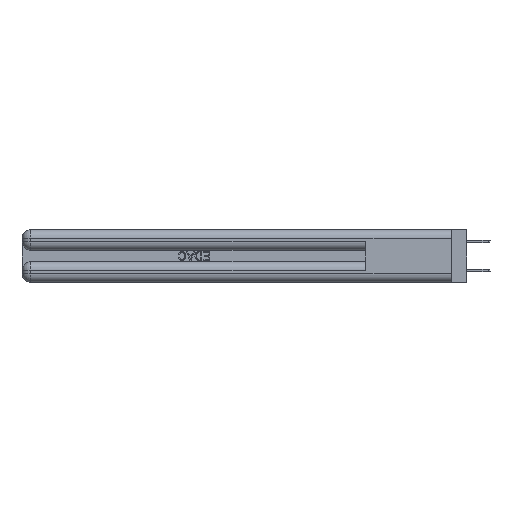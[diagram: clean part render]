
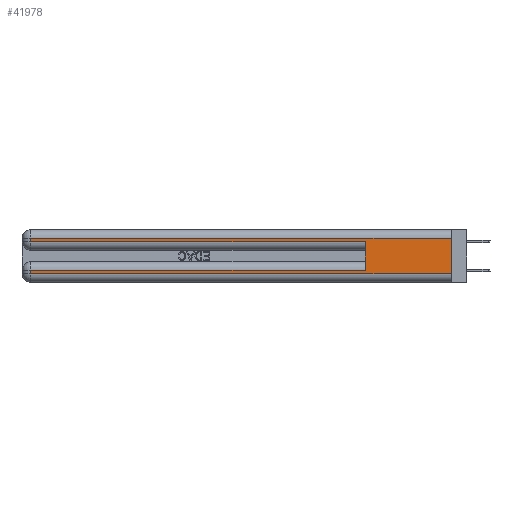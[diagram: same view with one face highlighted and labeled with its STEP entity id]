
A CAD part, left-side view. The second image highlights one B-rep face of the part: STEP entity #41978.
In plain terms, the highlighted planar face has unit normal (-1, 0, 0).
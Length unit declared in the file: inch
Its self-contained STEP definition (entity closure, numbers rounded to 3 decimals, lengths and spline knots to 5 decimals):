
#437 = DIRECTION ( 'NONE',  ( 0., 1., 0. ) ) ;
#550 = EDGE_CURVE ( 'NONE', #6409, #12220, #38957, .T. ) ;
#805 = LINE ( 'NONE', #17639, #45307 ) ;
#3940 = VECTOR ( 'NONE', #19840, 39.37008 ) ;
#4874 = CARTESIAN_POINT ( 'NONE',  ( 0., 0., 0.06 ) ) ;
#4940 = FACE_OUTER_BOUND ( 'NONE', #13955, .T. ) ;
#5453 = ORIENTED_EDGE ( 'NONE', *, *, #22547, .F. ) ;
#5785 = LINE ( 'NONE', #35403, #41984 ) ;
#6293 = DIRECTION ( 'NONE',  ( 0., 1., 0. ) ) ;
#6409 = VERTEX_POINT ( 'NONE', #10281 ) ;
#7810 = VERTEX_POINT ( 'NONE', #4874 ) ;
#7811 = PLANE ( 'NONE',  #12736 ) ;
#8340 = EDGE_CURVE ( 'NONE', #20547, #34211, #5785, .T. ) ;
#8510 = ORIENTED_EDGE ( 'NONE', *, *, #25732, .T. ) ;
#9078 = VERTEX_POINT ( 'NONE', #32416 ) ;
#9186 = LINE ( 'NONE', #11735, #33883 ) ;
#9234 = EDGE_CURVE ( 'NONE', #9078, #27472, #27751, .T. ) ;
#9552 = VECTOR ( 'NONE', #19166, 39.37008 ) ;
#10281 = CARTESIAN_POINT ( 'NONE',  ( 0., 0.6, 0.085 ) ) ;
#11735 = CARTESIAN_POINT ( 'NONE',  ( 0., 2.94, 0.37 ) ) ;
#12220 = VERTEX_POINT ( 'NONE', #26976 ) ;
#12345 = ORIENTED_EDGE ( 'NONE', *, *, #8340, .T. ) ;
#12736 = AXIS2_PLACEMENT_3D ( 'NONE', #14619, #39388, #18491 ) ;
#13955 = EDGE_LOOP ( 'NONE', ( #5453, #12345, #8510, #20647, #45182, #41907, #17926, #29409 ) ) ;
#14619 = CARTESIAN_POINT ( 'NONE',  ( 0., 0., 0.37 ) ) ;
#15609 = CARTESIAN_POINT ( 'NONE',  ( 0., 2.94, 0.37 ) ) ;
#17639 = CARTESIAN_POINT ( 'NONE',  ( 0., 0., 0.06 ) ) ;
#17926 = ORIENTED_EDGE ( 'NONE', *, *, #36855, .T. ) ;
#18491 = DIRECTION ( 'NONE',  ( 0., 0., -1. ) ) ;
#18560 = CARTESIAN_POINT ( 'NONE',  ( 0., 0., 0.37 ) ) ;
#19166 = DIRECTION ( 'NONE',  ( 0., 0., -1. ) ) ;
#19306 = DIRECTION ( 'NONE',  ( 0., -1., 0. ) ) ;
#19840 = DIRECTION ( 'NONE',  ( 0., 0., 1. ) ) ;
#20403 = VECTOR ( 'NONE', #6293, 39.37008 ) ;
#20459 = EDGE_CURVE ( 'NONE', #44820, #7810, #805, .T. ) ;
#20547 = VERTEX_POINT ( 'NONE', #21607 ) ;
#20647 = ORIENTED_EDGE ( 'NONE', *, *, #9234, .T. ) ;
#21158 = DIRECTION ( 'NONE',  ( 0., -1., 0. ) ) ;
#21528 = CARTESIAN_POINT ( 'NONE',  ( 0., 2.94, 0.06 ) ) ;
#21607 = CARTESIAN_POINT ( 'NONE',  ( 0., 0., 0.31 ) ) ;
#22547 = EDGE_CURVE ( 'NONE', #20547, #7810, #44561, .T. ) ;
#24910 = VECTOR ( 'NONE', #35960, 39.37008 ) ;
#25049 = CARTESIAN_POINT ( 'NONE',  ( 0., 0.6, 0.285 ) ) ;
#25732 = EDGE_CURVE ( 'NONE', #34211, #9078, #9186, .T. ) ;
#26976 = CARTESIAN_POINT ( 'NONE',  ( 0., 2.94, 0.085 ) ) ;
#27351 = CARTESIAN_POINT ( 'NONE',  ( 0., 0., 0.085 ) ) ;
#27472 = VERTEX_POINT ( 'NONE', #25049 ) ;
#27751 = LINE ( 'NONE', #43708, #37072 ) ;
#28239 = LINE ( 'NONE', #15609, #9552 ) ;
#29356 = DIRECTION ( 'NONE',  ( 0., 0., -1. ) ) ;
#29409 = ORIENTED_EDGE ( 'NONE', *, *, #20459, .T. ) ;
#32008 = LINE ( 'NONE', #33568, #3940 ) ;
#32416 = CARTESIAN_POINT ( 'NONE',  ( 0., 2.94, 0.285 ) ) ;
#33568 = CARTESIAN_POINT ( 'NONE',  ( 0., 0.6, 0.145 ) ) ;
#33883 = VECTOR ( 'NONE', #29356, 39.37008 ) ;
#34211 = VERTEX_POINT ( 'NONE', #39390 ) ;
#35403 = CARTESIAN_POINT ( 'NONE',  ( 0., 0., 0.31 ) ) ;
#35960 = DIRECTION ( 'NONE',  ( 0., 0., -1. ) ) ;
#36855 = EDGE_CURVE ( 'NONE', #12220, #44820, #28239, .T. ) ;
#37072 = VECTOR ( 'NONE', #19306, 39.37008 ) ;
#38957 = LINE ( 'NONE', #27351, #20403 ) ;
#39388 = DIRECTION ( 'NONE',  ( 1., 0., 0. ) ) ;
#39390 = CARTESIAN_POINT ( 'NONE',  ( 0., 2.94, 0.31 ) ) ;
#40652 = EDGE_CURVE ( 'NONE', #6409, #27472, #32008, .T. ) ;
#41907 = ORIENTED_EDGE ( 'NONE', *, *, #550, .T. ) ;
#41978 = ADVANCED_FACE ( 'NONE', ( #4940 ), #7811, .F. ) ;
#41984 = VECTOR ( 'NONE', #437, 39.37008 ) ;
#43708 = CARTESIAN_POINT ( 'NONE',  ( 0., 0., 0.285 ) ) ;
#44561 = LINE ( 'NONE', #18560, #24910 ) ;
#44820 = VERTEX_POINT ( 'NONE', #21528 ) ;
#45182 = ORIENTED_EDGE ( 'NONE', *, *, #40652, .F. ) ;
#45307 = VECTOR ( 'NONE', #21158, 39.37008 ) ;
